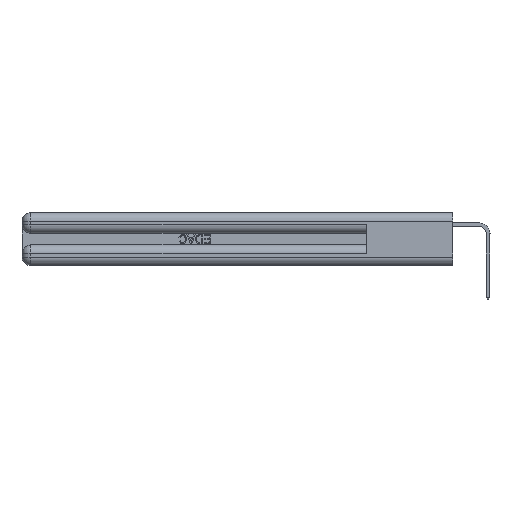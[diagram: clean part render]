
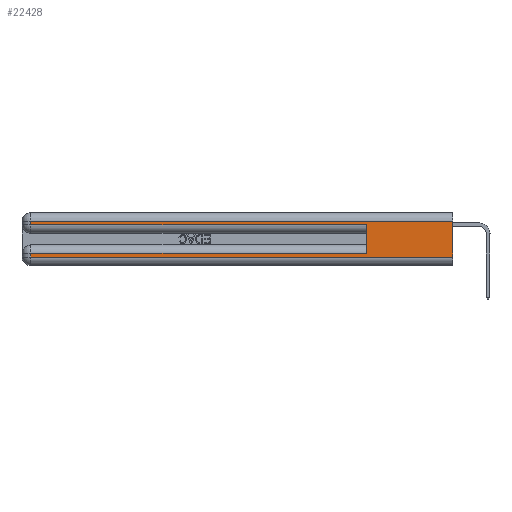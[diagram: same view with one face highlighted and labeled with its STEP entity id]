
A CAD part, left-side view. The second image highlights one B-rep face of the part: STEP entity #22428.
In plain terms, the highlighted planar face has unit normal (-1, 0, 0).
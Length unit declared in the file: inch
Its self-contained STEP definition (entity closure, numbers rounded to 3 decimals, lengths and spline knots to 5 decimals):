
#43 = EDGE_CURVE ( 'NONE', #15706, #23967, #13656, .T. ) ;
#239 = ORIENTED_EDGE ( 'NONE', *, *, #17752, .T. ) ;
#768 = VERTEX_POINT ( 'NONE', #40494 ) ;
#863 = ORIENTED_EDGE ( 'NONE', *, *, #33941, .F. ) ;
#2301 = VECTOR ( 'NONE', #47626, 39.37008 ) ;
#2517 = VERTEX_POINT ( 'NONE', #15676 ) ;
#3649 = CARTESIAN_POINT ( 'NONE',  ( 0., 2.94, 0.37 ) ) ;
#5196 = EDGE_CURVE ( 'NONE', #42265, #15706, #42902, .T. ) ;
#6799 = ORIENTED_EDGE ( 'NONE', *, *, #8096, .F. ) ;
#8096 = EDGE_CURVE ( 'NONE', #19567, #23967, #38820, .T. ) ;
#8207 = LINE ( 'NONE', #14907, #47354 ) ;
#8540 = LINE ( 'NONE', #3649, #18023 ) ;
#8959 = EDGE_LOOP ( 'NONE', ( #863, #239, #9169, #18136, #6799, #10630, #37762, #11357 ) ) ;
#9169 = ORIENTED_EDGE ( 'NONE', *, *, #5196, .T. ) ;
#10630 = ORIENTED_EDGE ( 'NONE', *, *, #42533, .T. ) ;
#10736 = VECTOR ( 'NONE', #49062, 39.37008 ) ;
#11357 = ORIENTED_EDGE ( 'NONE', *, *, #12981, .T. ) ;
#12981 = EDGE_CURVE ( 'NONE', #43474, #768, #8207, .T. ) ;
#13656 = LINE ( 'NONE', #27578, #33806 ) ;
#13925 = LINE ( 'NONE', #23988, #51696 ) ;
#14602 = PLANE ( 'NONE',  #35293 ) ;
#14907 = CARTESIAN_POINT ( 'NONE',  ( 0., 0., 0.06 ) ) ;
#15676 = CARTESIAN_POINT ( 'NONE',  ( 0., 2.94, 0.085 ) ) ;
#15706 = VERTEX_POINT ( 'NONE', #24996 ) ;
#17752 = EDGE_CURVE ( 'NONE', #43980, #42265, #38303, .T. ) ;
#18023 = VECTOR ( 'NONE', #23807, 39.37008 ) ;
#18136 = ORIENTED_EDGE ( 'NONE', *, *, #43, .T. ) ;
#18316 = CARTESIAN_POINT ( 'NONE',  ( 0., 0.6, 0.085 ) ) ;
#18640 = DIRECTION ( 'NONE',  ( 0., 0., -1. ) ) ;
#19105 = DIRECTION ( 'NONE',  ( 0., -1., 0. ) ) ;
#19377 = DIRECTION ( 'NONE',  ( 0., 0., 1. ) ) ;
#19567 = VERTEX_POINT ( 'NONE', #18316 ) ;
#22428 = ADVANCED_FACE ( 'NONE', ( #51758 ), #14602, .F. ) ;
#22575 = CARTESIAN_POINT ( 'NONE',  ( 0., 0., 0.31 ) ) ;
#23807 = DIRECTION ( 'NONE',  ( 0., 0., -1. ) ) ;
#23967 = VERTEX_POINT ( 'NONE', #39759 ) ;
#23988 = CARTESIAN_POINT ( 'NONE',  ( 0., 0., 0.085 ) ) ;
#24996 = CARTESIAN_POINT ( 'NONE',  ( 0., 2.94, 0.285 ) ) ;
#25094 = LINE ( 'NONE', #43568, #2301 ) ;
#25508 = EDGE_CURVE ( 'NONE', #2517, #43474, #8540, .T. ) ;
#27050 = DIRECTION ( 'NONE',  ( 0., -1., 0. ) ) ;
#27578 = CARTESIAN_POINT ( 'NONE',  ( 0., 0., 0.285 ) ) ;
#28037 = DIRECTION ( 'NONE',  ( 0., 1., 0. ) ) ;
#30642 = DIRECTION ( 'NONE',  ( 0., 1., 0. ) ) ;
#32388 = CARTESIAN_POINT ( 'NONE',  ( 0., 2.94, 0.06 ) ) ;
#33806 = VECTOR ( 'NONE', #19105, 39.37008 ) ;
#33941 = EDGE_CURVE ( 'NONE', #43980, #768, #25094, .T. ) ;
#34188 = CARTESIAN_POINT ( 'NONE',  ( 0., 2.94, 0.31 ) ) ;
#35293 = AXIS2_PLACEMENT_3D ( 'NONE', #50682, #42764, #18640 ) ;
#35383 = CARTESIAN_POINT ( 'NONE',  ( 0., 0.6, 0.145 ) ) ;
#37762 = ORIENTED_EDGE ( 'NONE', *, *, #25508, .T. ) ;
#38303 = LINE ( 'NONE', #22575, #46560 ) ;
#38820 = LINE ( 'NONE', #35383, #48330 ) ;
#39759 = CARTESIAN_POINT ( 'NONE',  ( 0., 0.6, 0.285 ) ) ;
#40231 = CARTESIAN_POINT ( 'NONE',  ( 0., 0., 0.31 ) ) ;
#40494 = CARTESIAN_POINT ( 'NONE',  ( 0., 0., 0.06 ) ) ;
#40924 = CARTESIAN_POINT ( 'NONE',  ( 0., 2.94, 0.37 ) ) ;
#42265 = VERTEX_POINT ( 'NONE', #34188 ) ;
#42533 = EDGE_CURVE ( 'NONE', #19567, #2517, #13925, .T. ) ;
#42764 = DIRECTION ( 'NONE',  ( 1., 0., 0. ) ) ;
#42902 = LINE ( 'NONE', #40924, #10736 ) ;
#43474 = VERTEX_POINT ( 'NONE', #32388 ) ;
#43568 = CARTESIAN_POINT ( 'NONE',  ( 0., 0., 0.37 ) ) ;
#43980 = VERTEX_POINT ( 'NONE', #40231 ) ;
#46560 = VECTOR ( 'NONE', #30642, 39.37008 ) ;
#47354 = VECTOR ( 'NONE', #27050, 39.37008 ) ;
#47626 = DIRECTION ( 'NONE',  ( 0., 0., -1. ) ) ;
#48330 = VECTOR ( 'NONE', #19377, 39.37008 ) ;
#49062 = DIRECTION ( 'NONE',  ( 0., 0., -1. ) ) ;
#50682 = CARTESIAN_POINT ( 'NONE',  ( 0., 0., 0.37 ) ) ;
#51696 = VECTOR ( 'NONE', #28037, 39.37008 ) ;
#51758 = FACE_OUTER_BOUND ( 'NONE', #8959, .T. ) ;
